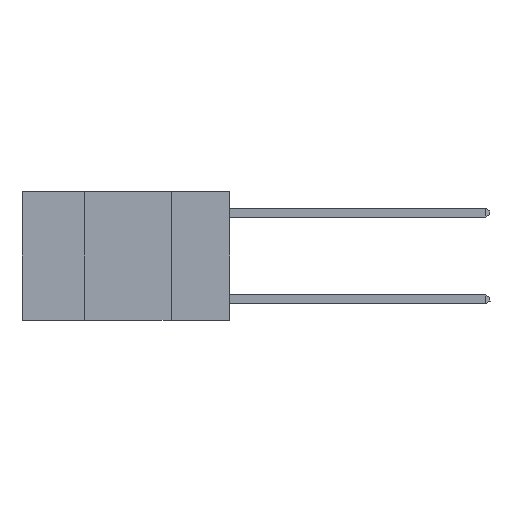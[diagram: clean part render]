
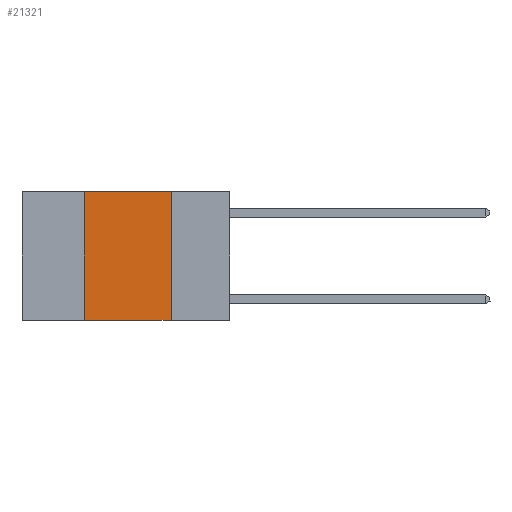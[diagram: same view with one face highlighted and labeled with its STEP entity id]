
A CAD part, left-side view. The second image highlights one B-rep face of the part: STEP entity #21321.
In plain terms, the highlighted planar face has unit normal (-1, 0, 0).
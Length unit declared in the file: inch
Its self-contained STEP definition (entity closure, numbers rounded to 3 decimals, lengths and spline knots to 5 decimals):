
#938 = VERTEX_POINT ( 'NONE', #15243 ) ;
#1498 = LINE ( 'NONE', #25311, #23164 ) ;
#1700 = VECTOR ( 'NONE', #6080, 39.37008 ) ;
#1882 = VECTOR ( 'NONE', #17132, 39.37008 ) ;
#2474 = ORIENTED_EDGE ( 'NONE', *, *, #25236, .F. ) ;
#3900 = CARTESIAN_POINT ( 'NONE',  ( 0., 0.6, -0.37 ) ) ;
#5149 = EDGE_CURVE ( 'NONE', #5654, #938, #23995, .T. ) ;
#5654 = VERTEX_POINT ( 'NONE', #12193 ) ;
#6080 = DIRECTION ( 'NONE',  ( 0., -1., 0. ) ) ;
#6243 = CARTESIAN_POINT ( 'NONE',  ( 0., 0.6, 0. ) ) ;
#6645 = CARTESIAN_POINT ( 'NONE',  ( 0., 0.17, 0. ) ) ;
#8646 = AXIS2_PLACEMENT_3D ( 'NONE', #6243, #24966, #12654 ) ;
#9878 = CARTESIAN_POINT ( 'NONE',  ( 0., 0.17, 0. ) ) ;
#10328 = EDGE_LOOP ( 'NONE', ( #11690, #11347, #2474, #12824 ) ) ;
#10527 = PLANE ( 'NONE',  #8646 ) ;
#10892 = EDGE_CURVE ( 'NONE', #25283, #938, #18760, .T. ) ;
#11347 = ORIENTED_EDGE ( 'NONE', *, *, #11630, .F. ) ;
#11630 = EDGE_CURVE ( 'NONE', #22441, #25283, #1498, .T. ) ;
#11690 = ORIENTED_EDGE ( 'NONE', *, *, #10892, .F. ) ;
#12193 = CARTESIAN_POINT ( 'NONE',  ( 0., 0.42, -0.37 ) ) ;
#12654 = DIRECTION ( 'NONE',  ( 0., 0., -1. ) ) ;
#12824 = ORIENTED_EDGE ( 'NONE', *, *, #5149, .T. ) ;
#15107 = DIRECTION ( 'NONE',  ( 0., -1., 0. ) ) ;
#15243 = CARTESIAN_POINT ( 'NONE',  ( 0., 0.17, -0.37 ) ) ;
#16026 = CARTESIAN_POINT ( 'NONE',  ( 0., 0.42, 0. ) ) ;
#17132 = DIRECTION ( 'NONE',  ( 0., 0., -1. ) ) ;
#18760 = LINE ( 'NONE', #6645, #1882 ) ;
#19225 = FACE_OUTER_BOUND ( 'NONE', #10328, .T. ) ;
#19350 = VECTOR ( 'NONE', #24264, 39.37008 ) ;
#19914 = CARTESIAN_POINT ( 'NONE',  ( 0., 0.42, 0. ) ) ;
#20005 = LINE ( 'NONE', #16026, #19350 ) ;
#21321 = ADVANCED_FACE ( 'NONE', ( #19225 ), #10527, .F. ) ;
#22441 = VERTEX_POINT ( 'NONE', #19914 ) ;
#23164 = VECTOR ( 'NONE', #15107, 39.37008 ) ;
#23995 = LINE ( 'NONE', #3900, #1700 ) ;
#24264 = DIRECTION ( 'NONE',  ( 0., 0., 1. ) ) ;
#24966 = DIRECTION ( 'NONE',  ( 1., 0., 0. ) ) ;
#25236 = EDGE_CURVE ( 'NONE', #5654, #22441, #20005, .T. ) ;
#25283 = VERTEX_POINT ( 'NONE', #9878 ) ;
#25311 = CARTESIAN_POINT ( 'NONE',  ( 0., 0.6, 0. ) ) ;
